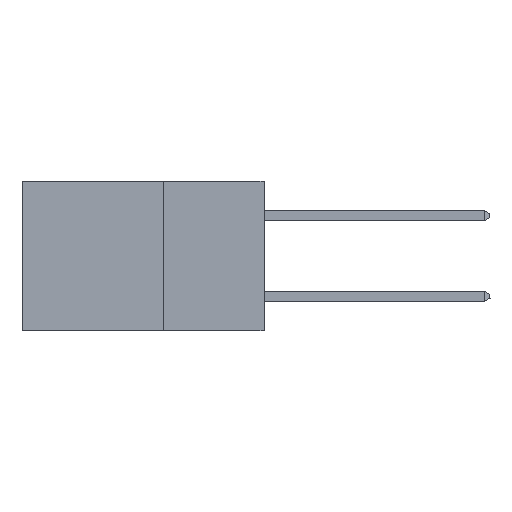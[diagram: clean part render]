
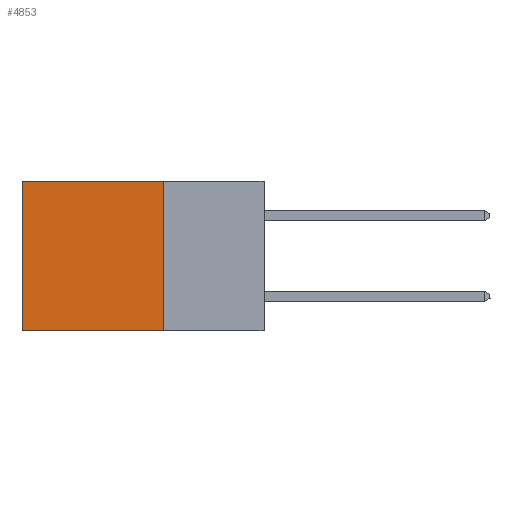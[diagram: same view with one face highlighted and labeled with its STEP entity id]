
A CAD part, left-side view. The second image highlights one B-rep face of the part: STEP entity #4853.
In plain terms, the highlighted planar face has unit normal (-1, 0, 0).
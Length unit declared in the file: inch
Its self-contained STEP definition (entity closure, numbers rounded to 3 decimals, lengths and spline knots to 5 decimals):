
#164 = ORIENTED_EDGE ( 'NONE', *, *, #6460, .F. ) ;
#619 = FACE_OUTER_BOUND ( 'NONE', #3642, .T. ) ;
#689 = ORIENTED_EDGE ( 'NONE', *, *, #9163, .T. ) ;
#2007 = CARTESIAN_POINT ( 'NONE',  ( 0.2615, 0.25, 0. ) ) ;
#2620 = VECTOR ( 'NONE', #2972, 39.37008 ) ;
#2719 = PLANE ( 'NONE',  #3284 ) ;
#2803 = EDGE_CURVE ( 'NONE', #3295, #9848, #6183, .T. ) ;
#2972 = DIRECTION ( 'NONE',  ( 0., 1., 0. ) ) ;
#3126 = ORIENTED_EDGE ( 'NONE', *, *, #5409, .F. ) ;
#3284 = AXIS2_PLACEMENT_3D ( 'NONE', #6772, #4275, #9745 ) ;
#3295 = VERTEX_POINT ( 'NONE', #6948 ) ;
#3588 = LINE ( 'NONE', #10074, #6750 ) ;
#3624 = LINE ( 'NONE', #8511, #4132 ) ;
#3642 = EDGE_LOOP ( 'NONE', ( #689, #3126, #164, #9850 ) ) ;
#4132 = VECTOR ( 'NONE', #7805, 39.37008 ) ;
#4275 = DIRECTION ( 'NONE',  ( 1., 0., 0. ) ) ;
#4294 = VERTEX_POINT ( 'NONE', #6466 ) ;
#4819 = CARTESIAN_POINT ( 'NONE',  ( 0.2615, 0.25, -0.37 ) ) ;
#4853 = ADVANCED_FACE ( 'NONE', ( #619 ), #2719, .F. ) ;
#4982 = LINE ( 'NONE', #5085, #5109 ) ;
#5085 = CARTESIAN_POINT ( 'NONE',  ( 0.2615, 0.25, -0.37 ) ) ;
#5109 = VECTOR ( 'NONE', #6665, 39.37008 ) ;
#5409 = EDGE_CURVE ( 'NONE', #8841, #4294, #4982, .T. ) ;
#6183 = LINE ( 'NONE', #2007, #2620 ) ;
#6214 = DIRECTION ( 'NONE',  ( 0., 0., -1. ) ) ;
#6460 = EDGE_CURVE ( 'NONE', #3295, #8841, #3624, .T. ) ;
#6466 = CARTESIAN_POINT ( 'NONE',  ( 0.2615, 0.6, -0.37 ) ) ;
#6665 = DIRECTION ( 'NONE',  ( 0., 1., 0. ) ) ;
#6750 = VECTOR ( 'NONE', #6214, 39.37008 ) ;
#6772 = CARTESIAN_POINT ( 'NONE',  ( 0.2615, 0.25, -0.37 ) ) ;
#6948 = CARTESIAN_POINT ( 'NONE',  ( 0.2615, 0.25, 0. ) ) ;
#7805 = DIRECTION ( 'NONE',  ( 0., 0., -1. ) ) ;
#8511 = CARTESIAN_POINT ( 'NONE',  ( 0.2615, 0.25, -0.37 ) ) ;
#8841 = VERTEX_POINT ( 'NONE', #4819 ) ;
#9163 = EDGE_CURVE ( 'NONE', #9848, #4294, #3588, .T. ) ;
#9380 = CARTESIAN_POINT ( 'NONE',  ( 0.2615, 0.6, 0. ) ) ;
#9745 = DIRECTION ( 'NONE',  ( 0., 0., -1. ) ) ;
#9848 = VERTEX_POINT ( 'NONE', #9380 ) ;
#9850 = ORIENTED_EDGE ( 'NONE', *, *, #2803, .T. ) ;
#10074 = CARTESIAN_POINT ( 'NONE',  ( 0.2615, 0.6, -0.37 ) ) ;
